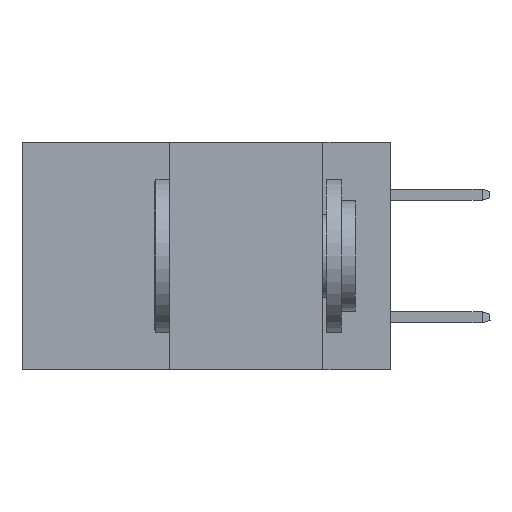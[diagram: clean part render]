
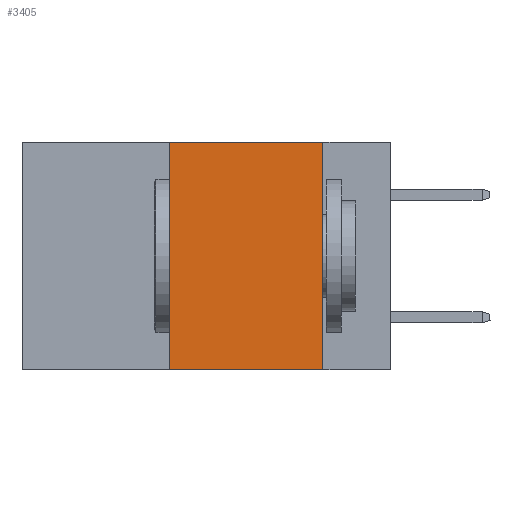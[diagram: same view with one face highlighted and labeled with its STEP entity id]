
A CAD part, left-side view. The second image highlights one B-rep face of the part: STEP entity #3405.
In plain terms, the highlighted planar face has unit normal (-1, 0, 0).
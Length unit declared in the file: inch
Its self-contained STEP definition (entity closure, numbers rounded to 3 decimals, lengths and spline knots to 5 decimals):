
#166 = EDGE_CURVE ( 'NONE', #6236, #8135, #11770, .T. ) ;
#329 = CARTESIAN_POINT ( 'NONE',  ( 0., 0.11, -0.37 ) ) ;
#2084 = ORIENTED_EDGE ( 'NONE', *, *, #166, .T. ) ;
#2619 = CARTESIAN_POINT ( 'NONE',  ( 0., 0.36, -0.37 ) ) ;
#2649 = CARTESIAN_POINT ( 'NONE',  ( 0., 0.6, 0. ) ) ;
#3405 = ADVANCED_FACE ( 'NONE', ( #5529 ), #5860, .F. ) ;
#3442 = ORIENTED_EDGE ( 'NONE', *, *, #4321, .F. ) ;
#3477 = DIRECTION ( 'NONE',  ( 0., -1., 0. ) ) ;
#4321 = EDGE_CURVE ( 'NONE', #6236, #5303, #8450, .T. ) ;
#4443 = VECTOR ( 'NONE', #9670, 39.37008 ) ;
#4464 = DIRECTION ( 'NONE',  ( 1., 0., 0. ) ) ;
#4475 = CARTESIAN_POINT ( 'NONE',  ( 0., 0.6, 0. ) ) ;
#4494 = ORIENTED_EDGE ( 'NONE', *, *, #4996, .F. ) ;
#4688 = CARTESIAN_POINT ( 'NONE',  ( 0., 0.6, -0.37 ) ) ;
#4996 = EDGE_CURVE ( 'NONE', #7793, #8135, #8072, .T. ) ;
#5303 = VERTEX_POINT ( 'NONE', #9752 ) ;
#5529 = FACE_OUTER_BOUND ( 'NONE', #10365, .T. ) ;
#5860 = PLANE ( 'NONE',  #9116 ) ;
#6236 = VERTEX_POINT ( 'NONE', #2619 ) ;
#6566 = VECTOR ( 'NONE', #3477, 39.37008 ) ;
#7793 = VERTEX_POINT ( 'NONE', #8970 ) ;
#8072 = LINE ( 'NONE', #12588, #12914 ) ;
#8135 = VERTEX_POINT ( 'NONE', #329 ) ;
#8165 = VECTOR ( 'NONE', #10389, 39.37008 ) ;
#8450 = LINE ( 'NONE', #10854, #8165 ) ;
#8970 = CARTESIAN_POINT ( 'NONE',  ( 0., 0.11, 0. ) ) ;
#9116 = AXIS2_PLACEMENT_3D ( 'NONE', #4475, #4464, #9947 ) ;
#9162 = ORIENTED_EDGE ( 'NONE', *, *, #12281, .F. ) ;
#9670 = DIRECTION ( 'NONE',  ( 0., -1., 0. ) ) ;
#9752 = CARTESIAN_POINT ( 'NONE',  ( 0., 0.36, 0. ) ) ;
#9947 = DIRECTION ( 'NONE',  ( 0., 0., -1. ) ) ;
#10365 = EDGE_LOOP ( 'NONE', ( #4494, #9162, #3442, #2084 ) ) ;
#10389 = DIRECTION ( 'NONE',  ( 0., 0., 1. ) ) ;
#10854 = CARTESIAN_POINT ( 'NONE',  ( 0., 0.36, 0. ) ) ;
#11770 = LINE ( 'NONE', #4688, #6566 ) ;
#12281 = EDGE_CURVE ( 'NONE', #5303, #7793, #12298, .T. ) ;
#12298 = LINE ( 'NONE', #2649, #4443 ) ;
#12583 = DIRECTION ( 'NONE',  ( 0., 0., -1. ) ) ;
#12588 = CARTESIAN_POINT ( 'NONE',  ( 0., 0.11, 0. ) ) ;
#12914 = VECTOR ( 'NONE', #12583, 39.37008 ) ;
